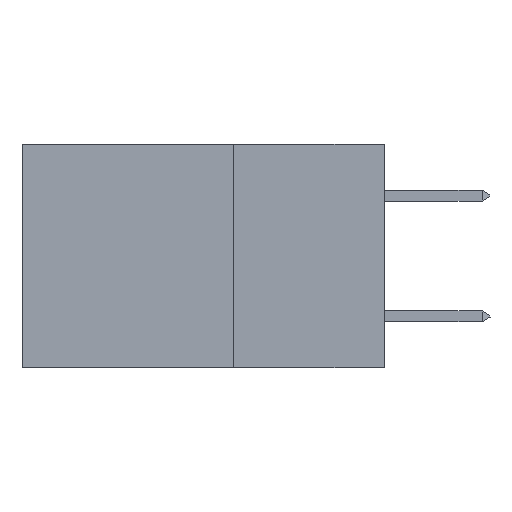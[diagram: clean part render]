
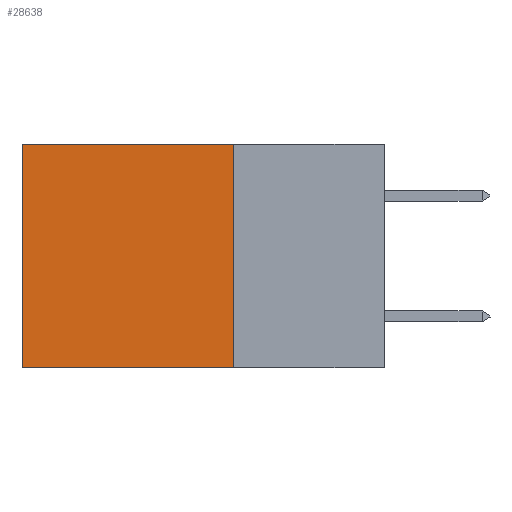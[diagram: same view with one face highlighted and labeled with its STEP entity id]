
A CAD part, left-side view. The second image highlights one B-rep face of the part: STEP entity #28638.
In plain terms, the highlighted planar face has unit normal (-1, 0, 0).
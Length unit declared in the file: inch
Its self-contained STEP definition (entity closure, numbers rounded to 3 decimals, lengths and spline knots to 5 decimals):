
#167 = VERTEX_POINT ( 'NONE', #24973 ) ;
#314 = DIRECTION ( 'NONE',  ( 0., 0., -1. ) ) ;
#1980 = EDGE_CURVE ( 'NONE', #167, #25883, #11389, .T. ) ;
#3026 = DIRECTION ( 'NONE',  ( 1., 0., 0. ) ) ;
#5621 = CARTESIAN_POINT ( 'NONE',  ( 0.2875, 0.6, 0. ) ) ;
#5760 = VERTEX_POINT ( 'NONE', #11313 ) ;
#7534 = CARTESIAN_POINT ( 'NONE',  ( 0.2875, 0.25, 0. ) ) ;
#9290 = DIRECTION ( 'NONE',  ( 0., 0., -1. ) ) ;
#9947 = DIRECTION ( 'NONE',  ( 0., 0., -1. ) ) ;
#10055 = PLANE ( 'NONE',  #28451 ) ;
#10254 = CARTESIAN_POINT ( 'NONE',  ( 0.2875, 0.6, 0. ) ) ;
#10424 = VECTOR ( 'NONE', #21974, 39.37008 ) ;
#11313 = CARTESIAN_POINT ( 'NONE',  ( 0.2875, 0.25, 0. ) ) ;
#11389 = LINE ( 'NONE', #16971, #14763 ) ;
#12115 = ORIENTED_EDGE ( 'NONE', *, *, #18586, .T. ) ;
#14549 = DIRECTION ( 'NONE',  ( 0., 1., 0. ) ) ;
#14763 = VECTOR ( 'NONE', #14549, 39.37008 ) ;
#16378 = CARTESIAN_POINT ( 'NONE',  ( 0.2875, 0.6, -0.37 ) ) ;
#16971 = CARTESIAN_POINT ( 'NONE',  ( 0.2875, 0.25, -0.37 ) ) ;
#18361 = VECTOR ( 'NONE', #9290, 39.37008 ) ;
#18586 = EDGE_CURVE ( 'NONE', #19994, #25883, #29609, .T. ) ;
#18969 = EDGE_CURVE ( 'NONE', #5760, #167, #22450, .T. ) ;
#19994 = VERTEX_POINT ( 'NONE', #5621 ) ;
#21974 = DIRECTION ( 'NONE',  ( 0., 1., 0. ) ) ;
#22450 = LINE ( 'NONE', #30590, #18361 ) ;
#24921 = ORIENTED_EDGE ( 'NONE', *, *, #1980, .F. ) ;
#24973 = CARTESIAN_POINT ( 'NONE',  ( 0.2875, 0.25, -0.37 ) ) ;
#25138 = EDGE_LOOP ( 'NONE', ( #12115, #24921, #28715, #26447 ) ) ;
#25883 = VERTEX_POINT ( 'NONE', #16378 ) ;
#26447 = ORIENTED_EDGE ( 'NONE', *, *, #30538, .T. ) ;
#26975 = VECTOR ( 'NONE', #314, 39.37008 ) ;
#27406 = FACE_OUTER_BOUND ( 'NONE', #25138, .T. ) ;
#28451 = AXIS2_PLACEMENT_3D ( 'NONE', #7534, #3026, #9947 ) ;
#28638 = ADVANCED_FACE ( 'NONE', ( #27406 ), #10055, .F. ) ;
#28715 = ORIENTED_EDGE ( 'NONE', *, *, #18969, .F. ) ;
#29308 = CARTESIAN_POINT ( 'NONE',  ( 0.2875, 0.25, 0. ) ) ;
#29609 = LINE ( 'NONE', #10254, #26975 ) ;
#30321 = LINE ( 'NONE', #29308, #10424 ) ;
#30538 = EDGE_CURVE ( 'NONE', #5760, #19994, #30321, .T. ) ;
#30590 = CARTESIAN_POINT ( 'NONE',  ( 0.2875, 0.25, 0. ) ) ;
